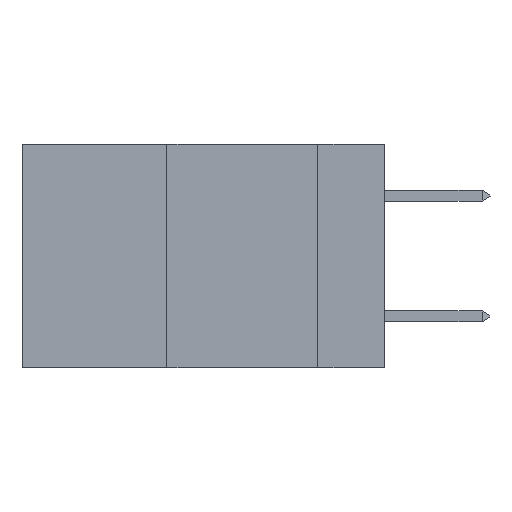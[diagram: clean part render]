
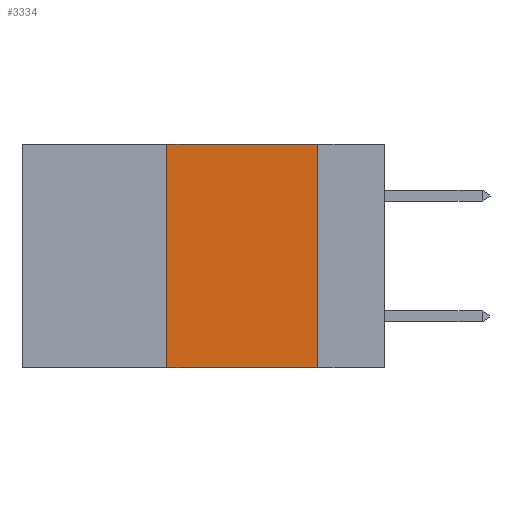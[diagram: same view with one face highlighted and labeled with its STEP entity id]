
A CAD part, left-side view. The second image highlights one B-rep face of the part: STEP entity #3334.
In plain terms, the highlighted planar face has unit normal (-1, 0, 0).
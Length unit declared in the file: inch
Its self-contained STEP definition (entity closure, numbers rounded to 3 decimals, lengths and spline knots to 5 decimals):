
#362 = CARTESIAN_POINT ( 'NONE',  ( 0., 0.36, -0.37 ) ) ;
#1175 = ORIENTED_EDGE ( 'NONE', *, *, #7154, .F. ) ;
#1331 = EDGE_CURVE ( 'NONE', #7293, #12239, #8913, .T. ) ;
#1516 = EDGE_CURVE ( 'NONE', #10537, #10663, #3774, .T. ) ;
#1896 = DIRECTION ( 'NONE',  ( 0., 0., 1. ) ) ;
#2470 = DIRECTION ( 'NONE',  ( 0., 0., -1. ) ) ;
#2844 = VECTOR ( 'NONE', #5634, 39.37008 ) ;
#2891 = CARTESIAN_POINT ( 'NONE',  ( 0., 0.11, -0.37 ) ) ;
#3159 = VECTOR ( 'NONE', #2470, 39.37008 ) ;
#3334 = ADVANCED_FACE ( 'NONE', ( #7178 ), #3987, .F. ) ;
#3774 = LINE ( 'NONE', #3847, #5709 ) ;
#3847 = CARTESIAN_POINT ( 'NONE',  ( 0., 0.6, -0.37 ) ) ;
#3987 = PLANE ( 'NONE',  #13257 ) ;
#4379 = EDGE_LOOP ( 'NONE', ( #1175, #6472, #6291, #6695 ) ) ;
#5634 = DIRECTION ( 'NONE',  ( 0., -1., 0. ) ) ;
#5709 = VECTOR ( 'NONE', #8311, 39.37008 ) ;
#6291 = ORIENTED_EDGE ( 'NONE', *, *, #9419, .F. ) ;
#6472 = ORIENTED_EDGE ( 'NONE', *, *, #1331, .F. ) ;
#6695 = ORIENTED_EDGE ( 'NONE', *, *, #1516, .T. ) ;
#7068 = CARTESIAN_POINT ( 'NONE',  ( 0., 0.11, 0. ) ) ;
#7154 = EDGE_CURVE ( 'NONE', #12239, #10663, #8140, .T. ) ;
#7178 = FACE_OUTER_BOUND ( 'NONE', #4379, .T. ) ;
#7293 = VERTEX_POINT ( 'NONE', #11663 ) ;
#7579 = CARTESIAN_POINT ( 'NONE',  ( 0., 0.36, 0. ) ) ;
#8140 = LINE ( 'NONE', #12722, #3159 ) ;
#8311 = DIRECTION ( 'NONE',  ( 0., -1., 0. ) ) ;
#8608 = LINE ( 'NONE', #7579, #14171 ) ;
#8913 = LINE ( 'NONE', #14623, #2844 ) ;
#9419 = EDGE_CURVE ( 'NONE', #10537, #7293, #8608, .T. ) ;
#9560 = DIRECTION ( 'NONE',  ( 1., 0., 0. ) ) ;
#9868 = CARTESIAN_POINT ( 'NONE',  ( 0., 0.6, 0. ) ) ;
#10537 = VERTEX_POINT ( 'NONE', #362 ) ;
#10663 = VERTEX_POINT ( 'NONE', #2891 ) ;
#11663 = CARTESIAN_POINT ( 'NONE',  ( 0., 0.36, 0. ) ) ;
#12239 = VERTEX_POINT ( 'NONE', #7068 ) ;
#12722 = CARTESIAN_POINT ( 'NONE',  ( 0., 0.11, 0. ) ) ;
#13257 = AXIS2_PLACEMENT_3D ( 'NONE', #9868, #9560, #14361 ) ;
#14171 = VECTOR ( 'NONE', #1896, 39.37008 ) ;
#14361 = DIRECTION ( 'NONE',  ( 0., 0., -1. ) ) ;
#14623 = CARTESIAN_POINT ( 'NONE',  ( 0., 0.6, 0. ) ) ;
